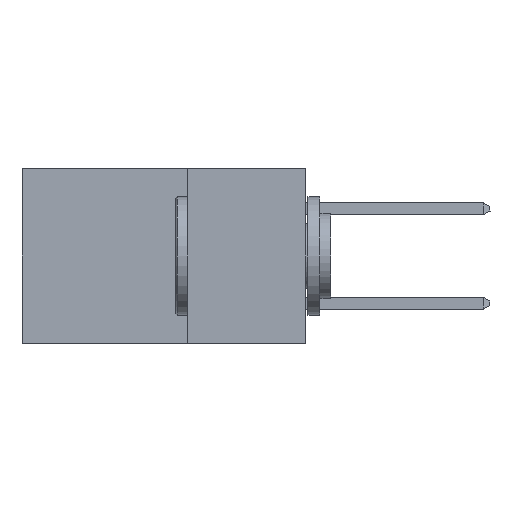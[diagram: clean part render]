
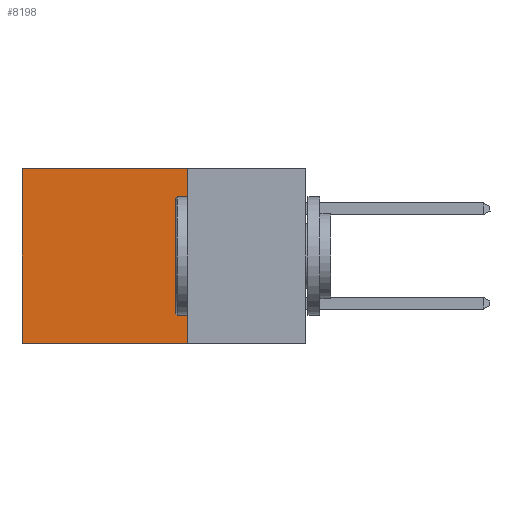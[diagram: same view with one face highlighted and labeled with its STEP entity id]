
A CAD part, left-side view. The second image highlights one B-rep face of the part: STEP entity #8198.
In plain terms, the highlighted planar face has unit normal (-1, 0, 0).
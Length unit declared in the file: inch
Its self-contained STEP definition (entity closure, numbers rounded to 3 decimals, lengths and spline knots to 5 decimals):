
#139 = LINE ( 'NONE', #6716, #3722 ) ;
#370 = LINE ( 'NONE', #12324, #16554 ) ;
#910 = DIRECTION ( 'NONE',  ( 0., 0., -1. ) ) ;
#1051 = PLANE ( 'NONE',  #7459 ) ;
#1173 = VERTEX_POINT ( 'NONE', #7003 ) ;
#2534 = LINE ( 'NONE', #8693, #3261 ) ;
#2724 = CARTESIAN_POINT ( 'NONE',  ( 0.298, 0.25, 0. ) ) ;
#2727 = VERTEX_POINT ( 'NONE', #10322 ) ;
#3261 = VECTOR ( 'NONE', #5637, 39.37008 ) ;
#3722 = VECTOR ( 'NONE', #12842, 39.37008 ) ;
#4911 = FACE_OUTER_BOUND ( 'NONE', #6469, .T. ) ;
#5465 = VERTEX_POINT ( 'NONE', #6240 ) ;
#5626 = ORIENTED_EDGE ( 'NONE', *, *, #7678, .T. ) ;
#5637 = DIRECTION ( 'NONE',  ( 0., 0., -1. ) ) ;
#5769 = ORIENTED_EDGE ( 'NONE', *, *, #14729, .T. ) ;
#6240 = CARTESIAN_POINT ( 'NONE',  ( 0.298, 0.25, 0. ) ) ;
#6469 = EDGE_LOOP ( 'NONE', ( #5626, #16556, #19113, #5769 ) ) ;
#6716 = CARTESIAN_POINT ( 'NONE',  ( 0.298, 0.6, 0. ) ) ;
#7003 = CARTESIAN_POINT ( 'NONE',  ( 0.298, 0.6, 0. ) ) ;
#7096 = VECTOR ( 'NONE', #13675, 39.37008 ) ;
#7323 = VERTEX_POINT ( 'NONE', #8733 ) ;
#7459 = AXIS2_PLACEMENT_3D ( 'NONE', #2724, #14757, #910 ) ;
#7678 = EDGE_CURVE ( 'NONE', #1173, #2727, #139, .T. ) ;
#8198 = ADVANCED_FACE ( 'NONE', ( #4911 ), #1051, .F. ) ;
#8693 = CARTESIAN_POINT ( 'NONE',  ( 0.298, 0.25, 0. ) ) ;
#8733 = CARTESIAN_POINT ( 'NONE',  ( 0.298, 0.25, -0.37 ) ) ;
#10322 = CARTESIAN_POINT ( 'NONE',  ( 0.298, 0.6, -0.37 ) ) ;
#12324 = CARTESIAN_POINT ( 'NONE',  ( 0.298, 0.25, -0.37 ) ) ;
#12842 = DIRECTION ( 'NONE',  ( 0., 0., -1. ) ) ;
#13059 = LINE ( 'NONE', #18810, #7096 ) ;
#13675 = DIRECTION ( 'NONE',  ( 0., 1., 0. ) ) ;
#14729 = EDGE_CURVE ( 'NONE', #5465, #1173, #13059, .T. ) ;
#14757 = DIRECTION ( 'NONE',  ( 1., 0., 0. ) ) ;
#15958 = EDGE_CURVE ( 'NONE', #7323, #2727, #370, .T. ) ;
#16554 = VECTOR ( 'NONE', #16821, 39.37008 ) ;
#16556 = ORIENTED_EDGE ( 'NONE', *, *, #15958, .F. ) ;
#16821 = DIRECTION ( 'NONE',  ( 0., 1., 0. ) ) ;
#18810 = CARTESIAN_POINT ( 'NONE',  ( 0.298, 0.25, 0. ) ) ;
#19113 = ORIENTED_EDGE ( 'NONE', *, *, #19625, .F. ) ;
#19625 = EDGE_CURVE ( 'NONE', #5465, #7323, #2534, .T. ) ;
